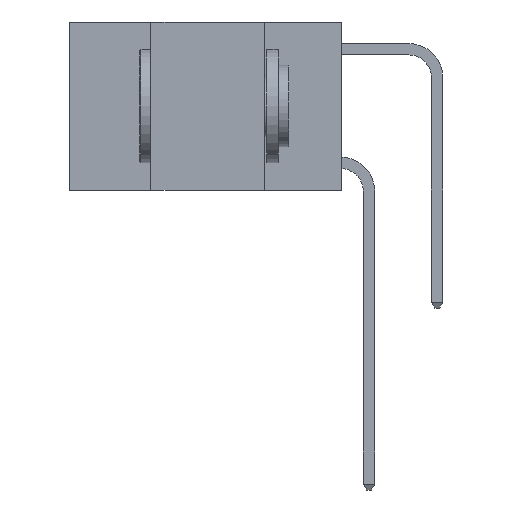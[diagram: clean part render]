
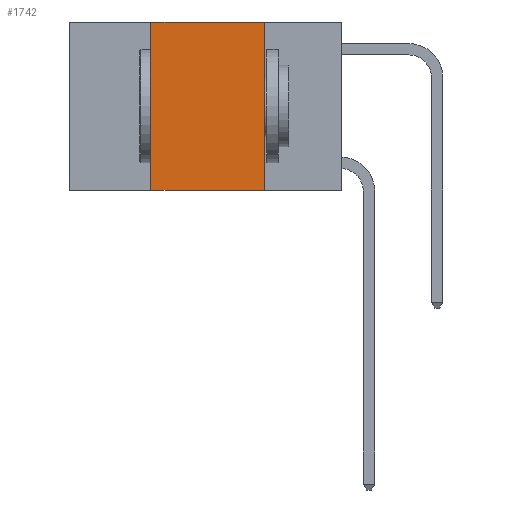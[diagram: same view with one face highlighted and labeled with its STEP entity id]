
A CAD part, left-side view. The second image highlights one B-rep face of the part: STEP entity #1742.
In plain terms, the highlighted planar face has unit normal (-1, 0, 0).
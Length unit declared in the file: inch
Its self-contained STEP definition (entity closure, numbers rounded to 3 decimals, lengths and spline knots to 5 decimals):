
#217 = DIRECTION ( 'NONE',  ( 0., -1., 0. ) ) ;
#499 = AXIS2_PLACEMENT_3D ( 'NONE', #5593, #2057, #8313 ) ;
#639 = EDGE_CURVE ( 'NONE', #11138, #1856, #10341, .T. ) ;
#1130 = ORIENTED_EDGE ( 'NONE', *, *, #10074, .F. ) ;
#1260 = CARTESIAN_POINT ( 'NONE',  ( 0., 0.6, -0.37 ) ) ;
#1319 = ORIENTED_EDGE ( 'NONE', *, *, #10753, .F. ) ;
#1345 = DIRECTION ( 'NONE',  ( 0., 0., -1. ) ) ;
#1742 = ADVANCED_FACE ( 'NONE', ( #9844 ), #6969, .F. ) ;
#1795 = VECTOR ( 'NONE', #1345, 39.37008 ) ;
#1856 = VERTEX_POINT ( 'NONE', #6395 ) ;
#2057 = DIRECTION ( 'NONE',  ( 1., 0., 0. ) ) ;
#2892 = LINE ( 'NONE', #1260, #5259 ) ;
#4536 = VERTEX_POINT ( 'NONE', #12223 ) ;
#4991 = VECTOR ( 'NONE', #7314, 39.37008 ) ;
#5259 = VECTOR ( 'NONE', #217, 39.37008 ) ;
#5593 = CARTESIAN_POINT ( 'NONE',  ( 0., 0.6, 0. ) ) ;
#6055 = ORIENTED_EDGE ( 'NONE', *, *, #12769, .T. ) ;
#6395 = CARTESIAN_POINT ( 'NONE',  ( 0., 0.17, 0. ) ) ;
#6969 = PLANE ( 'NONE',  #499 ) ;
#7314 = DIRECTION ( 'NONE',  ( 0., 0., 1. ) ) ;
#7317 = VECTOR ( 'NONE', #13004, 39.37008 ) ;
#7393 = CARTESIAN_POINT ( 'NONE',  ( 0., 0.17, 0. ) ) ;
#7981 = LINE ( 'NONE', #8347, #4991 ) ;
#7996 = VERTEX_POINT ( 'NONE', #8417 ) ;
#8134 = EDGE_LOOP ( 'NONE', ( #1319, #9880, #1130, #6055 ) ) ;
#8313 = DIRECTION ( 'NONE',  ( 0., 0., -1. ) ) ;
#8347 = CARTESIAN_POINT ( 'NONE',  ( 0., 0.42, 0. ) ) ;
#8417 = CARTESIAN_POINT ( 'NONE',  ( 0., 0.42, -0.37 ) ) ;
#9241 = CARTESIAN_POINT ( 'NONE',  ( 0., 0.6, 0. ) ) ;
#9844 = FACE_OUTER_BOUND ( 'NONE', #8134, .T. ) ;
#9880 = ORIENTED_EDGE ( 'NONE', *, *, #639, .F. ) ;
#10074 = EDGE_CURVE ( 'NONE', #7996, #11138, #7981, .T. ) ;
#10341 = LINE ( 'NONE', #9241, #7317 ) ;
#10753 = EDGE_CURVE ( 'NONE', #1856, #4536, #12221, .T. ) ;
#11138 = VERTEX_POINT ( 'NONE', #12124 ) ;
#12124 = CARTESIAN_POINT ( 'NONE',  ( 0., 0.42, 0. ) ) ;
#12221 = LINE ( 'NONE', #7393, #1795 ) ;
#12223 = CARTESIAN_POINT ( 'NONE',  ( 0., 0.17, -0.37 ) ) ;
#12769 = EDGE_CURVE ( 'NONE', #7996, #4536, #2892, .T. ) ;
#13004 = DIRECTION ( 'NONE',  ( 0., -1., 0. ) ) ;
